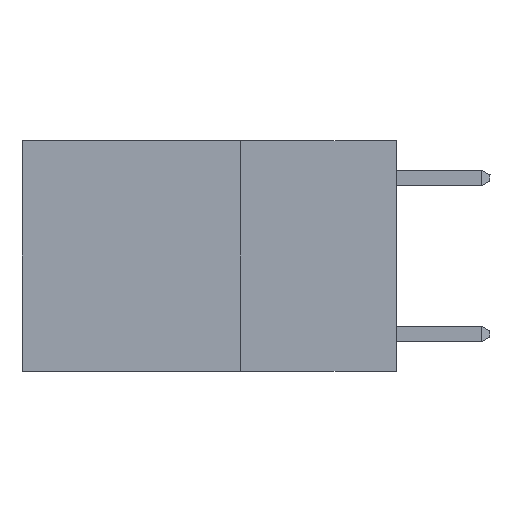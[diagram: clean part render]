
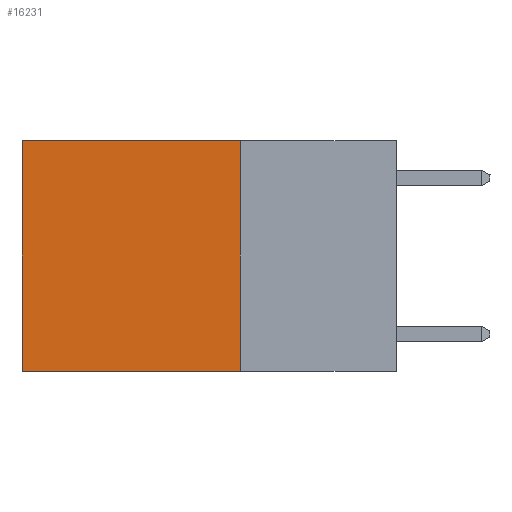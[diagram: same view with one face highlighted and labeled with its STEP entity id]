
A CAD part, left-side view. The second image highlights one B-rep face of the part: STEP entity #16231.
In plain terms, the highlighted planar face has unit normal (-1, 0, 0).
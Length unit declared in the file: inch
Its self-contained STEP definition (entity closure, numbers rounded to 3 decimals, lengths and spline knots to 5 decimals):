
#214 = DIRECTION ( 'NONE',  ( 0., 1., 0. ) ) ;
#1170 = CARTESIAN_POINT ( 'NONE',  ( 0.2625, 0.25, 0. ) ) ;
#1602 = ORIENTED_EDGE ( 'NONE', *, *, #15874, .T. ) ;
#2215 = CARTESIAN_POINT ( 'NONE',  ( 0.2625, 0.25, -0.37 ) ) ;
#2963 = EDGE_CURVE ( 'NONE', #15844, #17269, #10265, .T. ) ;
#3723 = VECTOR ( 'NONE', #214, 39.37008 ) ;
#4868 = EDGE_CURVE ( 'NONE', #9091, #17269, #18009, .T. ) ;
#4869 = AXIS2_PLACEMENT_3D ( 'NONE', #1170, #18158, #18250 ) ;
#4882 = VERTEX_POINT ( 'NONE', #11251 ) ;
#5152 = CARTESIAN_POINT ( 'NONE',  ( 0.2625, 0.6, 0. ) ) ;
#5835 = CARTESIAN_POINT ( 'NONE',  ( 0.2625, 0.25, 0. ) ) ;
#5965 = ORIENTED_EDGE ( 'NONE', *, *, #2963, .F. ) ;
#6822 = CARTESIAN_POINT ( 'NONE',  ( 0.2625, 0.25, 0. ) ) ;
#7039 = VECTOR ( 'NONE', #8069, 39.37008 ) ;
#7120 = CARTESIAN_POINT ( 'NONE',  ( 0.2625, 0.6, 0. ) ) ;
#7958 = LINE ( 'NONE', #6822, #9974 ) ;
#8069 = DIRECTION ( 'NONE',  ( 0., 0., -1. ) ) ;
#8595 = CARTESIAN_POINT ( 'NONE',  ( 0.2625, 0.6, -0.37 ) ) ;
#9091 = VERTEX_POINT ( 'NONE', #7120 ) ;
#9868 = ORIENTED_EDGE ( 'NONE', *, *, #13894, .F. ) ;
#9974 = VECTOR ( 'NONE', #12539, 39.37008 ) ;
#10055 = ORIENTED_EDGE ( 'NONE', *, *, #4868, .T. ) ;
#10157 = LINE ( 'NONE', #5835, #10205 ) ;
#10205 = VECTOR ( 'NONE', #18525, 39.37008 ) ;
#10265 = LINE ( 'NONE', #12029, #3723 ) ;
#11251 = CARTESIAN_POINT ( 'NONE',  ( 0.2625, 0.25, 0. ) ) ;
#12029 = CARTESIAN_POINT ( 'NONE',  ( 0.2625, 0.25, -0.37 ) ) ;
#12150 = PLANE ( 'NONE',  #4869 ) ;
#12539 = DIRECTION ( 'NONE',  ( 0., 1., 0. ) ) ;
#13894 = EDGE_CURVE ( 'NONE', #4882, #15844, #10157, .T. ) ;
#15844 = VERTEX_POINT ( 'NONE', #2215 ) ;
#15874 = EDGE_CURVE ( 'NONE', #4882, #9091, #7958, .T. ) ;
#16231 = ADVANCED_FACE ( 'NONE', ( #17966 ), #12150, .F. ) ;
#17269 = VERTEX_POINT ( 'NONE', #8595 ) ;
#17732 = EDGE_LOOP ( 'NONE', ( #10055, #5965, #9868, #1602 ) ) ;
#17966 = FACE_OUTER_BOUND ( 'NONE', #17732, .T. ) ;
#18009 = LINE ( 'NONE', #5152, #7039 ) ;
#18158 = DIRECTION ( 'NONE',  ( 1., 0., 0. ) ) ;
#18250 = DIRECTION ( 'NONE',  ( 0., 0., -1. ) ) ;
#18525 = DIRECTION ( 'NONE',  ( 0., 0., -1. ) ) ;
